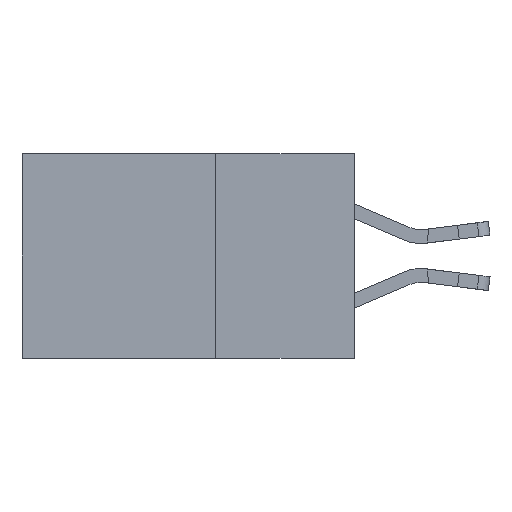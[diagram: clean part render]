
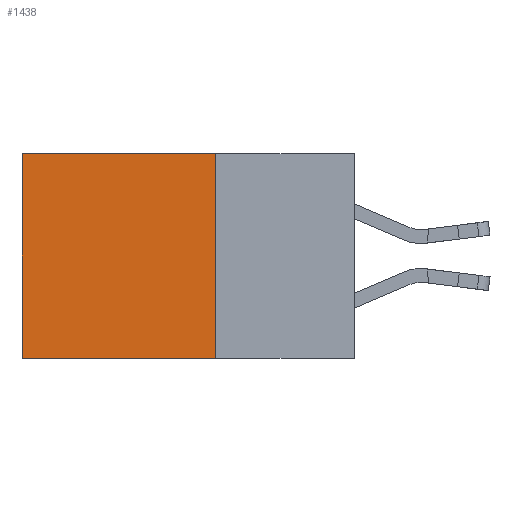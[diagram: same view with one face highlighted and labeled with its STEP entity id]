
A CAD part, left-side view. The second image highlights one B-rep face of the part: STEP entity #1438.
In plain terms, the highlighted planar face has unit normal (-1, 0, 0).
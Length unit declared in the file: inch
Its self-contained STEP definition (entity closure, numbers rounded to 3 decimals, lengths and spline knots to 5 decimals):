
#1010 = DIRECTION ( 'NONE',  ( 0., 1., 0. ) ) ;
#1438 = ADVANCED_FACE ( 'NONE', ( #3137 ), #3804, .F. ) ;
#1677 = VERTEX_POINT ( 'NONE', #20524 ) ;
#3137 = FACE_OUTER_BOUND ( 'NONE', #9854, .T. ) ;
#3804 = PLANE ( 'NONE',  #20858 ) ;
#4147 = VECTOR ( 'NONE', #10204, 39.37008 ) ;
#4941 = DIRECTION ( 'NONE',  ( 0., 0., -1. ) ) ;
#5037 = CARTESIAN_POINT ( 'NONE',  ( 0.298, 0.6, 0. ) ) ;
#8048 = EDGE_CURVE ( 'NONE', #15757, #1677, #8945, .T. ) ;
#8945 = LINE ( 'NONE', #16525, #16103 ) ;
#9250 = EDGE_CURVE ( 'NONE', #18053, #1677, #20263, .T. ) ;
#9340 = CARTESIAN_POINT ( 'NONE',  ( 0.298, 0.25, -0.37 ) ) ;
#9854 = EDGE_LOOP ( 'NONE', ( #12890, #15517, #15010, #20956 ) ) ;
#10204 = DIRECTION ( 'NONE',  ( 0., 0., -1. ) ) ;
#12890 = ORIENTED_EDGE ( 'NONE', *, *, #9250, .T. ) ;
#14693 = LINE ( 'NONE', #15969, #15471 ) ;
#15010 = ORIENTED_EDGE ( 'NONE', *, *, #20779, .F. ) ;
#15471 = VECTOR ( 'NONE', #20891, 39.37008 ) ;
#15490 = DIRECTION ( 'NONE',  ( 0., 0., -1. ) ) ;
#15517 = ORIENTED_EDGE ( 'NONE', *, *, #8048, .F. ) ;
#15757 = VERTEX_POINT ( 'NONE', #9340 ) ;
#15969 = CARTESIAN_POINT ( 'NONE',  ( 0.298, 0.25, 0. ) ) ;
#16103 = VECTOR ( 'NONE', #1010, 39.37008 ) ;
#16164 = EDGE_CURVE ( 'NONE', #20726, #18053, #14693, .T. ) ;
#16525 = CARTESIAN_POINT ( 'NONE',  ( 0.298, 0.25, -0.37 ) ) ;
#16611 = LINE ( 'NONE', #16632, #17260 ) ;
#16632 = CARTESIAN_POINT ( 'NONE',  ( 0.298, 0.25, 0. ) ) ;
#17125 = CARTESIAN_POINT ( 'NONE',  ( 0.298, 0.25, 0. ) ) ;
#17260 = VECTOR ( 'NONE', #4941, 39.37008 ) ;
#18053 = VERTEX_POINT ( 'NONE', #20003 ) ;
#20003 = CARTESIAN_POINT ( 'NONE',  ( 0.298, 0.6, 0. ) ) ;
#20263 = LINE ( 'NONE', #5037, #4147 ) ;
#20481 = DIRECTION ( 'NONE',  ( 1., 0., 0. ) ) ;
#20524 = CARTESIAN_POINT ( 'NONE',  ( 0.298, 0.6, -0.37 ) ) ;
#20678 = CARTESIAN_POINT ( 'NONE',  ( 0.298, 0.25, 0. ) ) ;
#20726 = VERTEX_POINT ( 'NONE', #20678 ) ;
#20779 = EDGE_CURVE ( 'NONE', #20726, #15757, #16611, .T. ) ;
#20858 = AXIS2_PLACEMENT_3D ( 'NONE', #17125, #20481, #15490 ) ;
#20891 = DIRECTION ( 'NONE',  ( 0., 1., 0. ) ) ;
#20956 = ORIENTED_EDGE ( 'NONE', *, *, #16164, .T. ) ;
